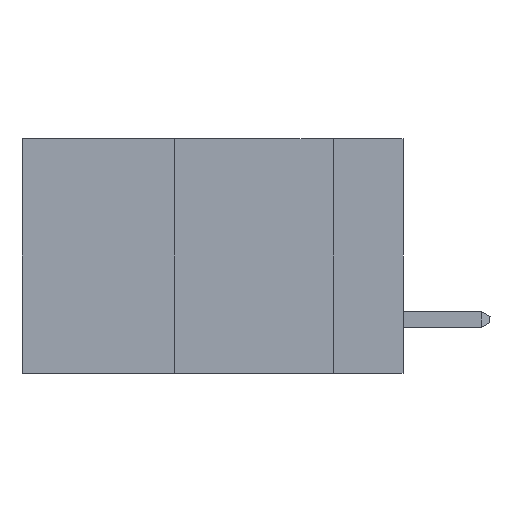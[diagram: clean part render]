
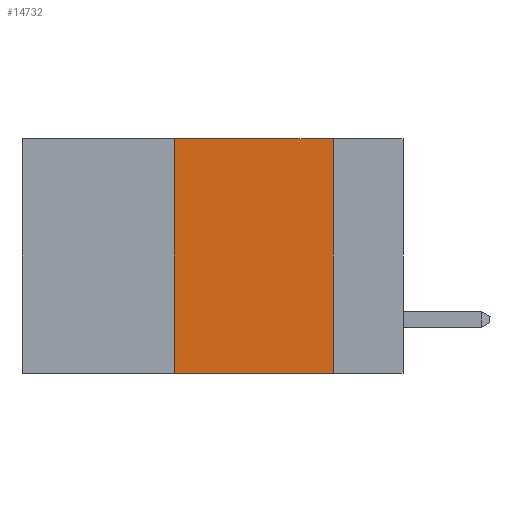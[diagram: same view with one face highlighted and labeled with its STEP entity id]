
A CAD part, left-side view. The second image highlights one B-rep face of the part: STEP entity #14732.
In plain terms, the highlighted planar face has unit normal (-1, 0, 0).
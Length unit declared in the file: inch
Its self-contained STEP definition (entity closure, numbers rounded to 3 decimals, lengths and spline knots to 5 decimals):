
#2853 = EDGE_CURVE ( 'NONE', #23708, #17966, #23573, .T. ) ;
#3559 = CARTESIAN_POINT ( 'NONE',  ( 0., 0.11, 0. ) ) ;
#5788 = EDGE_CURVE ( 'NONE', #23708, #25180, #10725, .T. ) ;
#5947 = ORIENTED_EDGE ( 'NONE', *, *, #16025, .F. ) ;
#6321 = ORIENTED_EDGE ( 'NONE', *, *, #2853, .T. ) ;
#6330 = FACE_OUTER_BOUND ( 'NONE', #22212, .T. ) ;
#7095 = DIRECTION ( 'NONE',  ( 0., -1., 0. ) ) ;
#8318 = DIRECTION ( 'NONE',  ( 0., -1., 0. ) ) ;
#9761 = CARTESIAN_POINT ( 'NONE',  ( 0., 0.36, 0. ) ) ;
#10538 = VECTOR ( 'NONE', #8318, 39.37008 ) ;
#10590 = PLANE ( 'NONE',  #31334 ) ;
#10725 = LINE ( 'NONE', #9761, #29494 ) ;
#12590 = EDGE_CURVE ( 'NONE', #13404, #17966, #27922, .T. ) ;
#13114 = VECTOR ( 'NONE', #7095, 39.37008 ) ;
#13404 = VERTEX_POINT ( 'NONE', #3559 ) ;
#14014 = DIRECTION ( 'NONE',  ( 0., 0., -1. ) ) ;
#14367 = DIRECTION ( 'NONE',  ( 0., 0., 1. ) ) ;
#14510 = VECTOR ( 'NONE', #14014, 39.37008 ) ;
#14732 = ADVANCED_FACE ( 'NONE', ( #6330 ), #10590, .F. ) ;
#15267 = ORIENTED_EDGE ( 'NONE', *, *, #5788, .F. ) ;
#16025 = EDGE_CURVE ( 'NONE', #25180, #13404, #16956, .T. ) ;
#16248 = ORIENTED_EDGE ( 'NONE', *, *, #12590, .F. ) ;
#16945 = CARTESIAN_POINT ( 'NONE',  ( 0., 0.6, 0. ) ) ;
#16956 = LINE ( 'NONE', #16945, #13114 ) ;
#17782 = DIRECTION ( 'NONE',  ( 1., 0., 0. ) ) ;
#17966 = VERTEX_POINT ( 'NONE', #20997 ) ;
#20997 = CARTESIAN_POINT ( 'NONE',  ( 0., 0.11, -0.37 ) ) ;
#21002 = DIRECTION ( 'NONE',  ( 0., 0., -1. ) ) ;
#22212 = EDGE_LOOP ( 'NONE', ( #16248, #5947, #15267, #6321 ) ) ;
#23573 = LINE ( 'NONE', #30358, #10538 ) ;
#23708 = VERTEX_POINT ( 'NONE', #27159 ) ;
#24405 = CARTESIAN_POINT ( 'NONE',  ( 0., 0.36, 0. ) ) ;
#25133 = CARTESIAN_POINT ( 'NONE',  ( 0., 0.6, 0. ) ) ;
#25180 = VERTEX_POINT ( 'NONE', #24405 ) ;
#27159 = CARTESIAN_POINT ( 'NONE',  ( 0., 0.36, -0.37 ) ) ;
#27922 = LINE ( 'NONE', #30898, #14510 ) ;
#29494 = VECTOR ( 'NONE', #14367, 39.37008 ) ;
#30358 = CARTESIAN_POINT ( 'NONE',  ( 0., 0.6, -0.37 ) ) ;
#30898 = CARTESIAN_POINT ( 'NONE',  ( 0., 0.11, 0. ) ) ;
#31334 = AXIS2_PLACEMENT_3D ( 'NONE', #25133, #17782, #21002 ) ;
